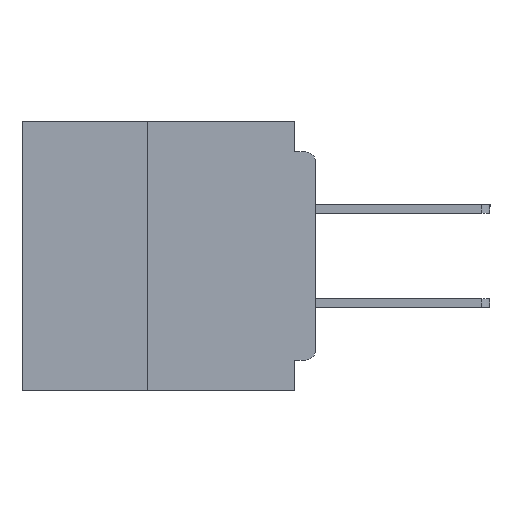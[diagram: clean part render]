
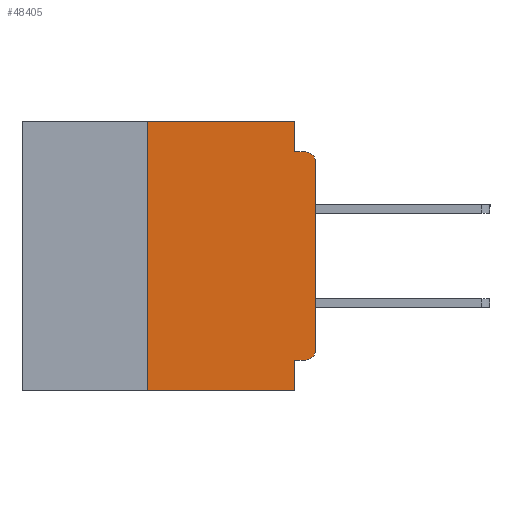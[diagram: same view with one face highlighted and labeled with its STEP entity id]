
A CAD part, left-side view. The second image highlights one B-rep face of the part: STEP entity #48405.
In plain terms, the highlighted planar face has unit normal (-1, 0, 0).
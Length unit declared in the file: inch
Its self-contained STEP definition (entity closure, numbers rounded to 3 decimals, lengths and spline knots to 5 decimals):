
#782 = EDGE_CURVE ( 'NONE', #21928, #45692, #5364, .T. ) ;
#895 = AXIS2_PLACEMENT_3D ( 'NONE', #62889, #32859, #2861 ) ;
#995 = ORIENTED_EDGE ( 'NONE', *, *, #2200, .F. ) ;
#1106 = CARTESIAN_POINT ( 'NONE',  ( 0., 0.437, -0.4 ) ) ;
#1155 = VECTOR ( 'NONE', #59887, 39.37008 ) ;
#2200 = EDGE_CURVE ( 'NONE', #59410, #17377, #27795, .T. ) ;
#2311 = VECTOR ( 'NONE', #21096, 39.37008 ) ;
#2861 = DIRECTION ( 'NONE',  ( 0., 0., -1. ) ) ;
#3729 = LINE ( 'NONE', #11151, #14009 ) ;
#4692 = ORIENTED_EDGE ( 'NONE', *, *, #782, .F. ) ;
#5364 = LINE ( 'NONE', #15151, #57081 ) ;
#5979 = EDGE_CURVE ( 'NONE', #46786, #28658, #17286, .T. ) ;
#6330 = CARTESIAN_POINT ( 'NONE',  ( 0., 0.25, -0.4 ) ) ;
#7808 = VECTOR ( 'NONE', #32277, 39.37008 ) ;
#8015 = ORIENTED_EDGE ( 'NONE', *, *, #57908, .T. ) ;
#8619 = CARTESIAN_POINT ( 'NONE',  ( 0., 0., -0.045 ) ) ;
#11151 = CARTESIAN_POINT ( 'NONE',  ( 0., 0., 0. ) ) ;
#12764 = EDGE_CURVE ( 'NONE', #17377, #28658, #25609, .T. ) ;
#13687 = DIRECTION ( 'NONE',  ( 0., -1., 0. ) ) ;
#14009 = VECTOR ( 'NONE', #36251, 39.37008 ) ;
#14340 = PLANE ( 'NONE',  #30577 ) ;
#15151 = CARTESIAN_POINT ( 'NONE',  ( 0., 0.437, 0. ) ) ;
#15357 = DIRECTION ( 'NONE',  ( 0., -1., 0. ) ) ;
#15457 = CIRCLE ( 'NONE', #895, 0.015 ) ;
#15934 = CARTESIAN_POINT ( 'NONE',  ( 0., 0.031, 0. ) ) ;
#16183 = EDGE_LOOP ( 'NONE', ( #42488, #8015, #32230, #47580, #4692, #42332, #16369, #44604, #995, #19776 ) ) ;
#16369 = ORIENTED_EDGE ( 'NONE', *, *, #5979, .T. ) ;
#17286 = LINE ( 'NONE', #1106, #2311 ) ;
#17377 = VERTEX_POINT ( 'NONE', #35518 ) ;
#18818 = VECTOR ( 'NONE', #13687, 39.37008 ) ;
#19342 = CARTESIAN_POINT ( 'NONE',  ( 0., 0.437, 0. ) ) ;
#19776 = ORIENTED_EDGE ( 'NONE', *, *, #42209, .T. ) ;
#20953 = DIRECTION ( 'NONE',  ( 0., 0., -1. ) ) ;
#21096 = DIRECTION ( 'NONE',  ( 0., -1., 0. ) ) ;
#21928 = VERTEX_POINT ( 'NONE', #53815 ) ;
#24333 = DIRECTION ( 'NONE',  ( 1., 0., 0. ) ) ;
#24409 = LINE ( 'NONE', #15934, #61209 ) ;
#24467 = CARTESIAN_POINT ( 'NONE',  ( 0., 0.031, -0.4 ) ) ;
#25600 = CARTESIAN_POINT ( 'NONE',  ( 0., 0.015, -0.045 ) ) ;
#25609 = LINE ( 'NONE', #50901, #62425 ) ;
#27658 = DIRECTION ( 'NONE',  ( -1., 0., 0. ) ) ;
#27795 = LINE ( 'NONE', #59588, #1155 ) ;
#28658 = VERTEX_POINT ( 'NONE', #24467 ) ;
#30577 = AXIS2_PLACEMENT_3D ( 'NONE', #19342, #24333, #59359 ) ;
#32230 = ORIENTED_EDGE ( 'NONE', *, *, #64369, .F. ) ;
#32277 = DIRECTION ( 'NONE',  ( 0., 0., 1. ) ) ;
#32859 = DIRECTION ( 'NONE',  ( -1., 0., 0. ) ) ;
#32961 = VERTEX_POINT ( 'NONE', #59079 ) ;
#35518 = CARTESIAN_POINT ( 'NONE',  ( 0., 0.031, -0.355 ) ) ;
#36251 = DIRECTION ( 'NONE',  ( 0., 0., 1. ) ) ;
#37884 = VERTEX_POINT ( 'NONE', #46161 ) ;
#41378 = EDGE_CURVE ( 'NONE', #32961, #37884, #3729, .T. ) ;
#42209 = EDGE_CURVE ( 'NONE', #59410, #32961, #15457, .T. ) ;
#42233 = LINE ( 'NONE', #8619, #18818 ) ;
#42332 = ORIENTED_EDGE ( 'NONE', *, *, #50649, .F. ) ;
#42488 = ORIENTED_EDGE ( 'NONE', *, *, #41378, .T. ) ;
#43142 = AXIS2_PLACEMENT_3D ( 'NONE', #57659, #27658, #62722 ) ;
#44604 = ORIENTED_EDGE ( 'NONE', *, *, #12764, .F. ) ;
#45596 = VERTEX_POINT ( 'NONE', #25600 ) ;
#45615 = FACE_OUTER_BOUND ( 'NONE', #16183, .T. ) ;
#45692 = VERTEX_POINT ( 'NONE', #56238 ) ;
#46161 = CARTESIAN_POINT ( 'NONE',  ( 0., 0., -0.06 ) ) ;
#46786 = VERTEX_POINT ( 'NONE', #6330 ) ;
#47580 = ORIENTED_EDGE ( 'NONE', *, *, #55941, .F. ) ;
#47746 = LINE ( 'NONE', #52243, #7808 ) ;
#48405 = ADVANCED_FACE ( 'NONE', ( #45615 ), #14340, .F. ) ;
#50649 = EDGE_CURVE ( 'NONE', #46786, #21928, #47746, .T. ) ;
#50901 = CARTESIAN_POINT ( 'NONE',  ( 0., 0.031, -0.4 ) ) ;
#51505 = CARTESIAN_POINT ( 'NONE',  ( 0., 0.015, -0.355 ) ) ;
#51993 = VERTEX_POINT ( 'NONE', #54255 ) ;
#52243 = CARTESIAN_POINT ( 'NONE',  ( 0., 0.25, -0.4 ) ) ;
#53815 = CARTESIAN_POINT ( 'NONE',  ( 0., 0.25, 0. ) ) ;
#54255 = CARTESIAN_POINT ( 'NONE',  ( 0., 0.031, -0.045 ) ) ;
#55941 = EDGE_CURVE ( 'NONE', #45692, #51993, #24409, .T. ) ;
#55949 = DIRECTION ( 'NONE',  ( 0., 0., -1. ) ) ;
#56238 = CARTESIAN_POINT ( 'NONE',  ( 0., 0.031, 0. ) ) ;
#57081 = VECTOR ( 'NONE', #15357, 39.37008 ) ;
#57659 = CARTESIAN_POINT ( 'NONE',  ( 0., 0.015, -0.06 ) ) ;
#57908 = EDGE_CURVE ( 'NONE', #37884, #45596, #63372, .T. ) ;
#59079 = CARTESIAN_POINT ( 'NONE',  ( 0., 0., -0.34 ) ) ;
#59359 = DIRECTION ( 'NONE',  ( 0., 0., -1. ) ) ;
#59410 = VERTEX_POINT ( 'NONE', #51505 ) ;
#59588 = CARTESIAN_POINT ( 'NONE',  ( 0., 0., -0.355 ) ) ;
#59887 = DIRECTION ( 'NONE',  ( 0., 1., 0. ) ) ;
#61209 = VECTOR ( 'NONE', #20953, 39.37008 ) ;
#62425 = VECTOR ( 'NONE', #55949, 39.37008 ) ;
#62722 = DIRECTION ( 'NONE',  ( 0., 0., -1. ) ) ;
#62889 = CARTESIAN_POINT ( 'NONE',  ( 0., 0.015, -0.34 ) ) ;
#63372 = CIRCLE ( 'NONE', #43142, 0.015 ) ;
#64369 = EDGE_CURVE ( 'NONE', #51993, #45596, #42233, .T. ) ;
